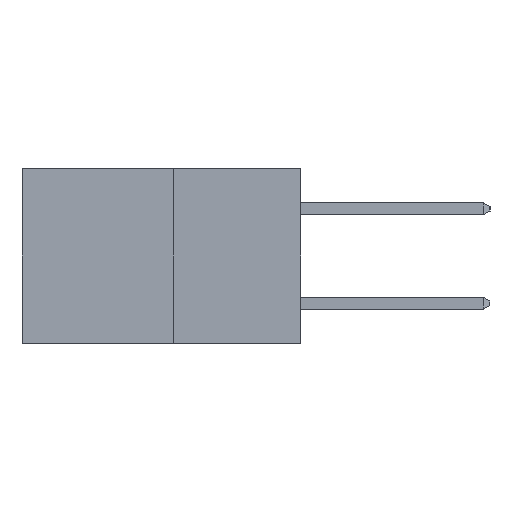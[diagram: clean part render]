
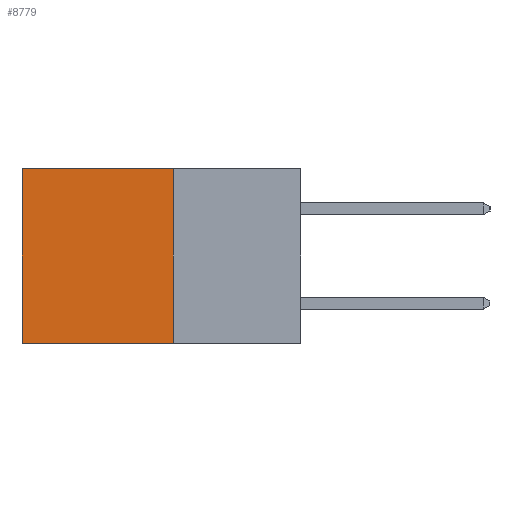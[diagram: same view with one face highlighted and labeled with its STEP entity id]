
A CAD part, left-side view. The second image highlights one B-rep face of the part: STEP entity #8779.
In plain terms, the highlighted planar face has unit normal (-1, 0, 0).
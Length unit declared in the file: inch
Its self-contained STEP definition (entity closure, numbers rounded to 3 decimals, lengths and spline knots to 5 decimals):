
#962 = ORIENTED_EDGE ( 'NONE', *, *, #7513, .F. ) ;
#1832 = EDGE_CURVE ( 'NONE', #3167, #10242, #3695, .T. ) ;
#2058 = PLANE ( 'NONE',  #4762 ) ;
#2528 = LINE ( 'NONE', #3778, #13215 ) ;
#3087 = LINE ( 'NONE', #6419, #13763 ) ;
#3167 = VERTEX_POINT ( 'NONE', #8535 ) ;
#3268 = VECTOR ( 'NONE', #13276, 39.37008 ) ;
#3422 = CARTESIAN_POINT ( 'NONE',  ( 0.277, 0.59, -0.37 ) ) ;
#3484 = DIRECTION ( 'NONE',  ( 0., 0., -1. ) ) ;
#3695 = LINE ( 'NONE', #13347, #3268 ) ;
#3778 = CARTESIAN_POINT ( 'NONE',  ( 0.277, 0.59, -0.37 ) ) ;
#3935 = CARTESIAN_POINT ( 'NONE',  ( 0.277, 0.27, -0.37 ) ) ;
#4762 = AXIS2_PLACEMENT_3D ( 'NONE', #15867, #11843, #3484 ) ;
#5176 = DIRECTION ( 'NONE',  ( 0., 0., -1. ) ) ;
#6419 = CARTESIAN_POINT ( 'NONE',  ( 0.277, 0.27, -0.37 ) ) ;
#6430 = VECTOR ( 'NONE', #6478, 39.37008 ) ;
#6478 = DIRECTION ( 'NONE',  ( 0., 0., -1. ) ) ;
#6864 = EDGE_CURVE ( 'NONE', #10242, #12106, #2528, .T. ) ;
#7513 = EDGE_CURVE ( 'NONE', #3167, #8312, #10154, .T. ) ;
#8230 = ORIENTED_EDGE ( 'NONE', *, *, #6864, .T. ) ;
#8312 = VERTEX_POINT ( 'NONE', #3935 ) ;
#8502 = ORIENTED_EDGE ( 'NONE', *, *, #1832, .T. ) ;
#8535 = CARTESIAN_POINT ( 'NONE',  ( 0.277, 0.27, 0. ) ) ;
#8779 = ADVANCED_FACE ( 'NONE', ( #8790 ), #2058, .F. ) ;
#8790 = FACE_OUTER_BOUND ( 'NONE', #12065, .T. ) ;
#10154 = LINE ( 'NONE', #16120, #6430 ) ;
#10239 = EDGE_CURVE ( 'NONE', #8312, #12106, #3087, .T. ) ;
#10242 = VERTEX_POINT ( 'NONE', #13369 ) ;
#11843 = DIRECTION ( 'NONE',  ( 1., 0., 0. ) ) ;
#12065 = EDGE_LOOP ( 'NONE', ( #8230, #15190, #962, #8502 ) ) ;
#12106 = VERTEX_POINT ( 'NONE', #3422 ) ;
#13215 = VECTOR ( 'NONE', #5176, 39.37008 ) ;
#13276 = DIRECTION ( 'NONE',  ( 0., 1., 0. ) ) ;
#13347 = CARTESIAN_POINT ( 'NONE',  ( 0.277, 0.27, 0. ) ) ;
#13369 = CARTESIAN_POINT ( 'NONE',  ( 0.277, 0.59, 0. ) ) ;
#13763 = VECTOR ( 'NONE', #16053, 39.37008 ) ;
#15190 = ORIENTED_EDGE ( 'NONE', *, *, #10239, .F. ) ;
#15867 = CARTESIAN_POINT ( 'NONE',  ( 0.277, 0.27, -0.37 ) ) ;
#16053 = DIRECTION ( 'NONE',  ( 0., 1., 0. ) ) ;
#16120 = CARTESIAN_POINT ( 'NONE',  ( 0.277, 0.27, -0.37 ) ) ;
